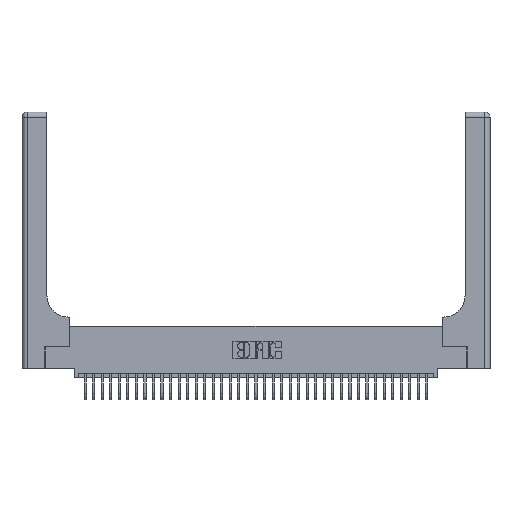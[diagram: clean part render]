
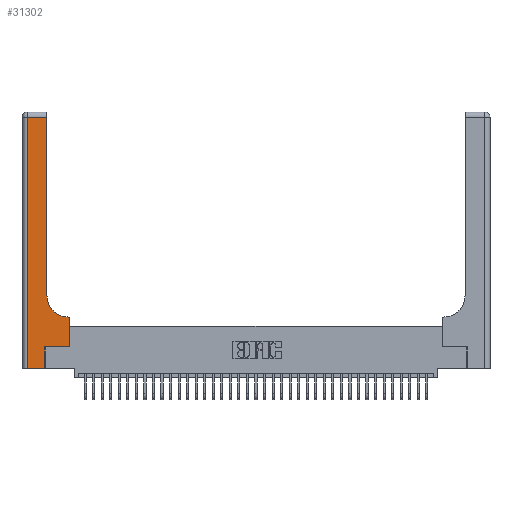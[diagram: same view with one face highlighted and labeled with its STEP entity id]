
A CAD part, top view. The second image highlights one B-rep face of the part: STEP entity #31302.
In plain terms, the highlighted planar face has unit normal (0, 0, 1).
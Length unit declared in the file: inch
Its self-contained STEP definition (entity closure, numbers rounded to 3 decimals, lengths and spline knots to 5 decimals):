
#204 = CARTESIAN_POINT ( 'NONE',  ( 0.269, 0.25, 0.37 ) ) ;
#536 = DIRECTION ( 'NONE',  ( -1., 0., 0. ) ) ;
#1510 = ORIENTED_EDGE ( 'NONE', *, *, #31649, .T. ) ;
#1625 = VECTOR ( 'NONE', #21503, 39.37008 ) ;
#1744 = EDGE_CURVE ( 'NONE', #31310, #16079, #25016, .T. ) ;
#2071 = CARTESIAN_POINT ( 'NONE',  ( 0.5585, 0.25, 0.37 ) ) ;
#2082 = DIRECTION ( 'NONE',  ( 0., 0., -1. ) ) ;
#2754 = CARTESIAN_POINT ( 'NONE',  ( 0.269, 0., 0.37 ) ) ;
#2791 = VECTOR ( 'NONE', #22511, 39.37008 ) ;
#3163 = LINE ( 'NONE', #12845, #24735 ) ;
#3481 = ORIENTED_EDGE ( 'NONE', *, *, #23647, .T. ) ;
#3771 = AXIS2_PLACEMENT_3D ( 'NONE', #33592, #17001, #36400 ) ;
#4017 = VECTOR ( 'NONE', #31218, 39.37008 ) ;
#4157 = VERTEX_POINT ( 'NONE', #2071 ) ;
#5688 = VECTOR ( 'NONE', #536, 39.37008 ) ;
#7344 = ORIENTED_EDGE ( 'NONE', *, *, #35103, .T. ) ;
#7763 = VECTOR ( 'NONE', #13391, 39.37008 ) ;
#7778 = CARTESIAN_POINT ( 'NONE',  ( 0.269, 0.25, 0.37 ) ) ;
#7999 = EDGE_CURVE ( 'NONE', #23074, #18711, #17573, .T. ) ;
#8541 = ORIENTED_EDGE ( 'NONE', *, *, #20969, .T. ) ;
#8677 = LINE ( 'NONE', #7778, #7763 ) ;
#9280 = ORIENTED_EDGE ( 'NONE', *, *, #11554, .T. ) ;
#9538 = LINE ( 'NONE', #2754, #2791 ) ;
#9650 = EDGE_CURVE ( 'NONE', #33432, #4157, #8677, .T. ) ;
#10553 = LINE ( 'NONE', #21225, #24473 ) ;
#11554 = EDGE_CURVE ( 'NONE', #18711, #36054, #10553, .T. ) ;
#12845 = CARTESIAN_POINT ( 'NONE',  ( 0.5585, 0.25, 0.37 ) ) ;
#13306 = LINE ( 'NONE', #17578, #5688 ) ;
#13391 = DIRECTION ( 'NONE',  ( 1., 0., 0. ) ) ;
#13608 = CARTESIAN_POINT ( 'NONE',  ( 0.06, 0., 0.37 ) ) ;
#15271 = CARTESIAN_POINT ( 'NONE',  ( 0., 0., 0.37 ) ) ;
#15934 = VECTOR ( 'NONE', #26166, 39.37008 ) ;
#16079 = VERTEX_POINT ( 'NONE', #33928 ) ;
#16258 = PLANE ( 'NONE',  #28291 ) ;
#17001 = DIRECTION ( 'NONE',  ( 0., 0., -1. ) ) ;
#17573 = CIRCLE ( 'NONE', #3771, 0.25 ) ;
#17578 = CARTESIAN_POINT ( 'NONE',  ( 0., 2.94, 0.37 ) ) ;
#17597 = ORIENTED_EDGE ( 'NONE', *, *, #7999, .T. ) ;
#17615 = CARTESIAN_POINT ( 'NONE',  ( 0.5585, 0.6, 0.37 ) ) ;
#18219 = CARTESIAN_POINT ( 'NONE',  ( 0.5415, 0.6, 0.37 ) ) ;
#18711 = VERTEX_POINT ( 'NONE', #23965 ) ;
#19668 = CARTESIAN_POINT ( 'NONE',  ( 0.06, 2.94, 0.37 ) ) ;
#20969 = EDGE_CURVE ( 'NONE', #22969, #23074, #26420, .T. ) ;
#21136 = DIRECTION ( 'NONE',  ( 0., 1., 0. ) ) ;
#21225 = CARTESIAN_POINT ( 'NONE',  ( 0.2915, 3., 0.37 ) ) ;
#21503 = DIRECTION ( 'NONE',  ( 1., 0., 0. ) ) ;
#21885 = DIRECTION ( 'NONE',  ( -1., 0., 0. ) ) ;
#22511 = DIRECTION ( 'NONE',  ( 0., 1., 0. ) ) ;
#22969 = VERTEX_POINT ( 'NONE', #17615 ) ;
#23074 = VERTEX_POINT ( 'NONE', #18219 ) ;
#23139 = ORIENTED_EDGE ( 'NONE', *, *, #9650, .T. ) ;
#23403 = CARTESIAN_POINT ( 'NONE',  ( 0.06, 3., 0.37 ) ) ;
#23647 = EDGE_CURVE ( 'NONE', #34021, #31310, #31580, .T. ) ;
#23965 = CARTESIAN_POINT ( 'NONE',  ( 0.2915, 0.85, 0.37 ) ) ;
#24473 = VECTOR ( 'NONE', #32336, 39.37008 ) ;
#24565 = ORIENTED_EDGE ( 'NONE', *, *, #29556, .T. ) ;
#24735 = VECTOR ( 'NONE', #21136, 39.37008 ) ;
#25016 = LINE ( 'NONE', #15271, #1625 ) ;
#26119 = ORIENTED_EDGE ( 'NONE', *, *, #1744, .T. ) ;
#26166 = DIRECTION ( 'NONE',  ( 0., -1., 0. ) ) ;
#26325 = FACE_OUTER_BOUND ( 'NONE', #27897, .T. ) ;
#26420 = LINE ( 'NONE', #28420, #4017 ) ;
#27897 = EDGE_LOOP ( 'NONE', ( #9280, #1510, #3481, #26119, #7344, #23139, #24565, #8541, #17597 ) ) ;
#28291 = AXIS2_PLACEMENT_3D ( 'NONE', #35665, #2082, #21885 ) ;
#28420 = CARTESIAN_POINT ( 'NONE',  ( 0.2915, 0.6, 0.37 ) ) ;
#29556 = EDGE_CURVE ( 'NONE', #4157, #22969, #3163, .T. ) ;
#31218 = DIRECTION ( 'NONE',  ( -1., 0., 0. ) ) ;
#31302 = ADVANCED_FACE ( 'NONE', ( #26325 ), #16258, .F. ) ;
#31310 = VERTEX_POINT ( 'NONE', #13608 ) ;
#31580 = LINE ( 'NONE', #23403, #15934 ) ;
#31649 = EDGE_CURVE ( 'NONE', #36054, #34021, #13306, .T. ) ;
#31710 = CARTESIAN_POINT ( 'NONE',  ( 0.2915, 2.94, 0.37 ) ) ;
#32336 = DIRECTION ( 'NONE',  ( 0., 1., 0. ) ) ;
#33432 = VERTEX_POINT ( 'NONE', #204 ) ;
#33592 = CARTESIAN_POINT ( 'NONE',  ( 0.5415, 0.85, 0.37 ) ) ;
#33928 = CARTESIAN_POINT ( 'NONE',  ( 0.269, 0., 0.37 ) ) ;
#34021 = VERTEX_POINT ( 'NONE', #19668 ) ;
#35103 = EDGE_CURVE ( 'NONE', #16079, #33432, #9538, .T. ) ;
#35665 = CARTESIAN_POINT ( 'NONE',  ( 0., 3., 0.37 ) ) ;
#36054 = VERTEX_POINT ( 'NONE', #31710 ) ;
#36400 = DIRECTION ( 'NONE',  ( 1., 0., 0. ) ) ;
